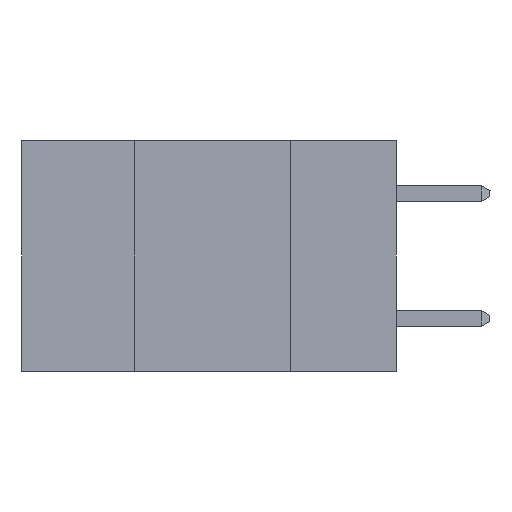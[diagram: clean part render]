
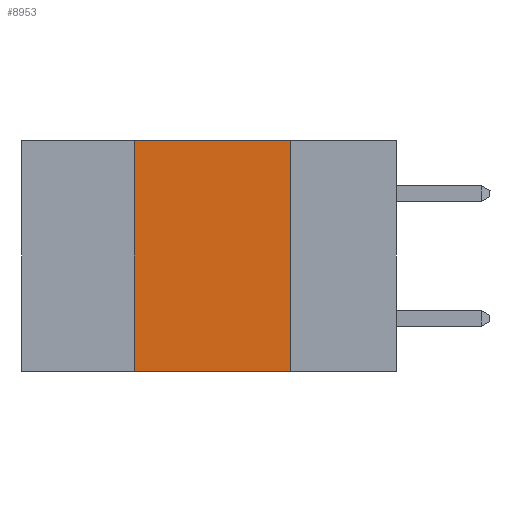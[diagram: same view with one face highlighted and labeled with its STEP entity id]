
A CAD part, left-side view. The second image highlights one B-rep face of the part: STEP entity #8953.
In plain terms, the highlighted planar face has unit normal (-1, 0, 0).
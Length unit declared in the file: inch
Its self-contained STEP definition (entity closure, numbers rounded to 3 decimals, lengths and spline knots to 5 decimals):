
#253 = VERTEX_POINT ( 'NONE', #6885 ) ;
#798 = CARTESIAN_POINT ( 'NONE',  ( 0., 0.6, 0. ) ) ;
#860 = LINE ( 'NONE', #961, #5804 ) ;
#961 = CARTESIAN_POINT ( 'NONE',  ( 0., 0.6, -0.37 ) ) ;
#1154 = CARTESIAN_POINT ( 'NONE',  ( 0., 0.6, 0. ) ) ;
#1322 = DIRECTION ( 'NONE',  ( 0., 0., -1. ) ) ;
#1673 = AXIS2_PLACEMENT_3D ( 'NONE', #798, #7656, #1818 ) ;
#1675 = CARTESIAN_POINT ( 'NONE',  ( 0., 0.42, -0.37 ) ) ;
#1818 = DIRECTION ( 'NONE',  ( 0., 0., -1. ) ) ;
#2190 = VERTEX_POINT ( 'NONE', #4345 ) ;
#2233 = VERTEX_POINT ( 'NONE', #1675 ) ;
#2363 = EDGE_CURVE ( 'NONE', #2233, #2430, #7150, .T. ) ;
#2430 = VERTEX_POINT ( 'NONE', #2505 ) ;
#2505 = CARTESIAN_POINT ( 'NONE',  ( 0., 0.42, 0. ) ) ;
#2601 = LINE ( 'NONE', #8175, #4944 ) ;
#3303 = EDGE_LOOP ( 'NONE', ( #12067, #4688, #9373, #6160 ) ) ;
#3835 = VECTOR ( 'NONE', #8980, 39.37008 ) ;
#4345 = CARTESIAN_POINT ( 'NONE',  ( 0., 0.17, -0.37 ) ) ;
#4688 = ORIENTED_EDGE ( 'NONE', *, *, #10751, .F. ) ;
#4944 = VECTOR ( 'NONE', #1322, 39.37008 ) ;
#5083 = FACE_OUTER_BOUND ( 'NONE', #3303, .T. ) ;
#5228 = CARTESIAN_POINT ( 'NONE',  ( 0., 0.42, 0. ) ) ;
#5804 = VECTOR ( 'NONE', #6854, 39.37008 ) ;
#6160 = ORIENTED_EDGE ( 'NONE', *, *, #7824, .T. ) ;
#6695 = PLANE ( 'NONE',  #1673 ) ;
#6854 = DIRECTION ( 'NONE',  ( 0., -1., 0. ) ) ;
#6885 = CARTESIAN_POINT ( 'NONE',  ( 0., 0.17, 0. ) ) ;
#7150 = LINE ( 'NONE', #5228, #10027 ) ;
#7656 = DIRECTION ( 'NONE',  ( 1., 0., 0. ) ) ;
#7824 = EDGE_CURVE ( 'NONE', #2233, #2190, #860, .T. ) ;
#8175 = CARTESIAN_POINT ( 'NONE',  ( 0., 0.17, 0. ) ) ;
#8726 = EDGE_CURVE ( 'NONE', #253, #2190, #2601, .T. ) ;
#8953 = ADVANCED_FACE ( 'NONE', ( #5083 ), #6695, .F. ) ;
#8980 = DIRECTION ( 'NONE',  ( 0., -1., 0. ) ) ;
#9022 = DIRECTION ( 'NONE',  ( 0., 0., 1. ) ) ;
#9373 = ORIENTED_EDGE ( 'NONE', *, *, #2363, .F. ) ;
#10027 = VECTOR ( 'NONE', #9022, 39.37008 ) ;
#10751 = EDGE_CURVE ( 'NONE', #2430, #253, #11514, .T. ) ;
#11514 = LINE ( 'NONE', #1154, #3835 ) ;
#12067 = ORIENTED_EDGE ( 'NONE', *, *, #8726, .F. ) ;
